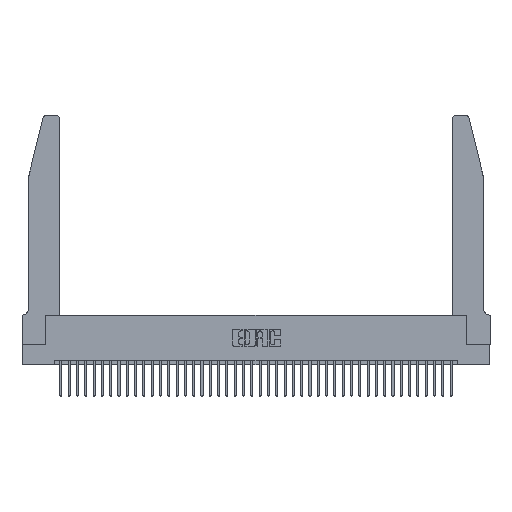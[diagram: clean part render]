
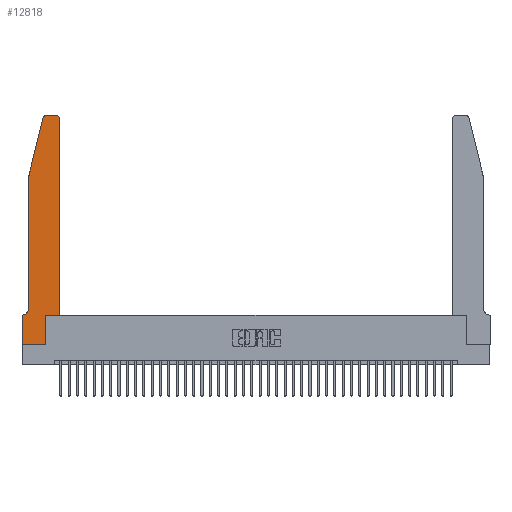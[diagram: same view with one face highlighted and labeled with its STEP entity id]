
A CAD part, top view. The second image highlights one B-rep face of the part: STEP entity #12818.
In plain terms, the highlighted planar face has unit normal (0, 0, 1).
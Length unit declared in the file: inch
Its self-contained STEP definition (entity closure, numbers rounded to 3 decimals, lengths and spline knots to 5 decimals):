
#75 = LINE ( 'NONE', #2907, #23874 ) ;
#559 = VERTEX_POINT ( 'NONE', #4509 ) ;
#716 = AXIS2_PLACEMENT_3D ( 'NONE', #13932, #36293, #17185 ) ;
#1324 = VERTEX_POINT ( 'NONE', #4705 ) ;
#1525 = DIRECTION ( 'NONE',  ( 1., 0., 0. ) ) ;
#1611 = VERTEX_POINT ( 'NONE', #41103 ) ;
#1766 = VECTOR ( 'NONE', #1525, 39.37008 ) ;
#2335 = LINE ( 'NONE', #2745, #18524 ) ;
#2400 = DIRECTION ( 'NONE',  ( -0.239, -0.971, 0. ) ) ;
#2684 = CIRCLE ( 'NONE', #11256, 0.03 ) ;
#2745 = CARTESIAN_POINT ( 'NONE',  ( 0.0755, 2., 0.37 ) ) ;
#2907 = CARTESIAN_POINT ( 'NONE',  ( 0.0755, 0.35, 0.37 ) ) ;
#3047 = CARTESIAN_POINT ( 'NONE',  ( 0.4505, 0.35, 0.37 ) ) ;
#3474 = EDGE_CURVE ( 'NONE', #559, #16719, #5469, .T. ) ;
#3603 = CARTESIAN_POINT ( 'NONE',  ( 0.0055, 0.42, 0.37 ) ) ;
#4028 = CARTESIAN_POINT ( 'NONE',  ( 0., 0.35, 0.37 ) ) ;
#4033 = VERTEX_POINT ( 'NONE', #35768 ) ;
#4509 = CARTESIAN_POINT ( 'NONE',  ( 0.25487, 2.72718, 0.37 ) ) ;
#4705 = CARTESIAN_POINT ( 'NONE',  ( 0.2865, 0., 0.37 ) ) ;
#4726 = EDGE_CURVE ( 'NONE', #26935, #1611, #10474, .T. ) ;
#4953 = CARTESIAN_POINT ( 'NONE',  ( 0.4505, 2.72, 0.37 ) ) ;
#5469 = LINE ( 'NONE', #15298, #38561 ) ;
#5759 = CARTESIAN_POINT ( 'NONE',  ( 0.2605, 2.75, 0.37 ) ) ;
#6904 = DIRECTION ( 'NONE',  ( -1., 0., 0. ) ) ;
#7255 = EDGE_CURVE ( 'NONE', #15617, #12796, #24191, .T. ) ;
#10474 = LINE ( 'NONE', #17711, #1766 ) ;
#10570 = DIRECTION ( 'NONE',  ( 1., 0., 0. ) ) ;
#10971 = EDGE_CURVE ( 'NONE', #36200, #29615, #38333, .T. ) ;
#11256 = AXIS2_PLACEMENT_3D ( 'NONE', #15887, #38200, #19076 ) ;
#11496 = EDGE_CURVE ( 'NONE', #27657, #559, #2684, .T. ) ;
#11683 = CARTESIAN_POINT ( 'NONE',  ( 0.2865, 0.35, 0.37 ) ) ;
#11935 = ORIENTED_EDGE ( 'NONE', *, *, #27538, .T. ) ;
#12314 = CARTESIAN_POINT ( 'NONE',  ( 0., 0.35, 0.37 ) ) ;
#12796 = VERTEX_POINT ( 'NONE', #23034 ) ;
#12818 = ADVANCED_FACE ( 'NONE', ( #19712 ), #23312, .T. ) ;
#13233 = ORIENTED_EDGE ( 'NONE', *, *, #4726, .T. ) ;
#13507 = VECTOR ( 'NONE', #41048, 39.37008 ) ;
#13932 = CARTESIAN_POINT ( 'NONE',  ( 0.4205, 2.72, 0.37 ) ) ;
#14524 = EDGE_CURVE ( 'NONE', #15896, #4033, #24140, .T. ) ;
#15131 = CARTESIAN_POINT ( 'NONE',  ( 0.2865, 0.35, 0.37 ) ) ;
#15138 = CARTESIAN_POINT ( 'NONE',  ( 0.0755, 2., 0.37 ) ) ;
#15298 = CARTESIAN_POINT ( 'NONE',  ( 0.0755, 2., 0.37 ) ) ;
#15617 = VERTEX_POINT ( 'NONE', #4953 ) ;
#15666 = ORIENTED_EDGE ( 'NONE', *, *, #3474, .T. ) ;
#15887 = CARTESIAN_POINT ( 'NONE',  ( 0.284, 2.72, 0.37 ) ) ;
#15896 = VERTEX_POINT ( 'NONE', #12314 ) ;
#16321 = VECTOR ( 'NONE', #27649, 39.37008 ) ;
#16667 = VECTOR ( 'NONE', #41449, 39.37008 ) ;
#16719 = VERTEX_POINT ( 'NONE', #15138 ) ;
#17185 = DIRECTION ( 'NONE',  ( 1., 0., 0. ) ) ;
#17212 = VECTOR ( 'NONE', #22363, 39.37008 ) ;
#17711 = CARTESIAN_POINT ( 'NONE',  ( 0.4505, 0.35, 0.37 ) ) ;
#18524 = VECTOR ( 'NONE', #28498, 39.37008 ) ;
#18759 = ORIENTED_EDGE ( 'NONE', *, *, #20614, .T. ) ;
#19076 = DIRECTION ( 'NONE',  ( 1., 0., 0. ) ) ;
#19140 = CARTESIAN_POINT ( 'NONE',  ( 0., 0., 0.37 ) ) ;
#19679 = CARTESIAN_POINT ( 'NONE',  ( 0.0755, 0.42, 0.37 ) ) ;
#19712 = FACE_OUTER_BOUND ( 'NONE', #22068, .T. ) ;
#20614 = EDGE_CURVE ( 'NONE', #16719, #36200, #2335, .T. ) ;
#21451 = AXIS2_PLACEMENT_3D ( 'NONE', #3603, #26097, #6904 ) ;
#21647 = ORIENTED_EDGE ( 'NONE', *, *, #7255, .T. ) ;
#22068 = EDGE_LOOP ( 'NONE', ( #26498, #25441, #15666, #18759, #32411, #11935, #27042, #22399, #37167, #13233, #39650, #21647 ) ) ;
#22363 = DIRECTION ( 'NONE',  ( 0., 1., 0. ) ) ;
#22399 = ORIENTED_EDGE ( 'NONE', *, *, #25178, .T. ) ;
#23034 = CARTESIAN_POINT ( 'NONE',  ( 0.4205, 2.75, 0.37 ) ) ;
#23312 = PLANE ( 'NONE',  #38865 ) ;
#23874 = VECTOR ( 'NONE', #28651, 39.37008 ) ;
#24137 = EDGE_CURVE ( 'NONE', #1324, #26935, #33279, .T. ) ;
#24140 = LINE ( 'NONE', #19140, #16667 ) ;
#24191 = CIRCLE ( 'NONE', #716, 0.03 ) ;
#24663 = LINE ( 'NONE', #3047, #17212 ) ;
#25178 = EDGE_CURVE ( 'NONE', #4033, #1324, #35701, .T. ) ;
#25441 = ORIENTED_EDGE ( 'NONE', *, *, #11496, .T. ) ;
#25737 = EDGE_CURVE ( 'NONE', #12796, #27657, #38994, .T. ) ;
#26097 = DIRECTION ( 'NONE',  ( 0., 0., -1. ) ) ;
#26498 = ORIENTED_EDGE ( 'NONE', *, *, #25737, .T. ) ;
#26935 = VERTEX_POINT ( 'NONE', #15131 ) ;
#27042 = ORIENTED_EDGE ( 'NONE', *, *, #14524, .T. ) ;
#27192 = VECTOR ( 'NONE', #35411, 39.37008 ) ;
#27538 = EDGE_CURVE ( 'NONE', #29615, #15896, #75, .T. ) ;
#27649 = DIRECTION ( 'NONE',  ( 0., 1., 0. ) ) ;
#27657 = VERTEX_POINT ( 'NONE', #34369 ) ;
#28498 = DIRECTION ( 'NONE',  ( 0., -1., 0. ) ) ;
#28651 = DIRECTION ( 'NONE',  ( -1., 0., 0. ) ) ;
#29615 = VERTEX_POINT ( 'NONE', #34379 ) ;
#29721 = DIRECTION ( 'NONE',  ( 0., 0., 1. ) ) ;
#29735 = EDGE_CURVE ( 'NONE', #1611, #15617, #24663, .T. ) ;
#32173 = CARTESIAN_POINT ( 'NONE',  ( 0., 0., 0.37 ) ) ;
#32411 = ORIENTED_EDGE ( 'NONE', *, *, #10971, .T. ) ;
#33279 = LINE ( 'NONE', #11683, #16321 ) ;
#34369 = CARTESIAN_POINT ( 'NONE',  ( 0.284, 2.75, 0.37 ) ) ;
#34379 = CARTESIAN_POINT ( 'NONE',  ( 0.0055, 0.35, 0.37 ) ) ;
#35411 = DIRECTION ( 'NONE',  ( 1., 0., 0. ) ) ;
#35701 = LINE ( 'NONE', #32173, #27192 ) ;
#35768 = CARTESIAN_POINT ( 'NONE',  ( 0., 0., 0.37 ) ) ;
#36200 = VERTEX_POINT ( 'NONE', #19679 ) ;
#36293 = DIRECTION ( 'NONE',  ( 0., 0., 1. ) ) ;
#37167 = ORIENTED_EDGE ( 'NONE', *, *, #24137, .T. ) ;
#38200 = DIRECTION ( 'NONE',  ( 0., 0., 1. ) ) ;
#38333 = CIRCLE ( 'NONE', #21451, 0.07 ) ;
#38561 = VECTOR ( 'NONE', #2400, 39.37008 ) ;
#38865 = AXIS2_PLACEMENT_3D ( 'NONE', #4028, #29721, #10570 ) ;
#38994 = LINE ( 'NONE', #5759, #13507 ) ;
#39650 = ORIENTED_EDGE ( 'NONE', *, *, #29735, .T. ) ;
#41048 = DIRECTION ( 'NONE',  ( -1., 0., 0. ) ) ;
#41103 = CARTESIAN_POINT ( 'NONE',  ( 0.4505, 0.35, 0.37 ) ) ;
#41449 = DIRECTION ( 'NONE',  ( 0., -1., 0. ) ) ;
